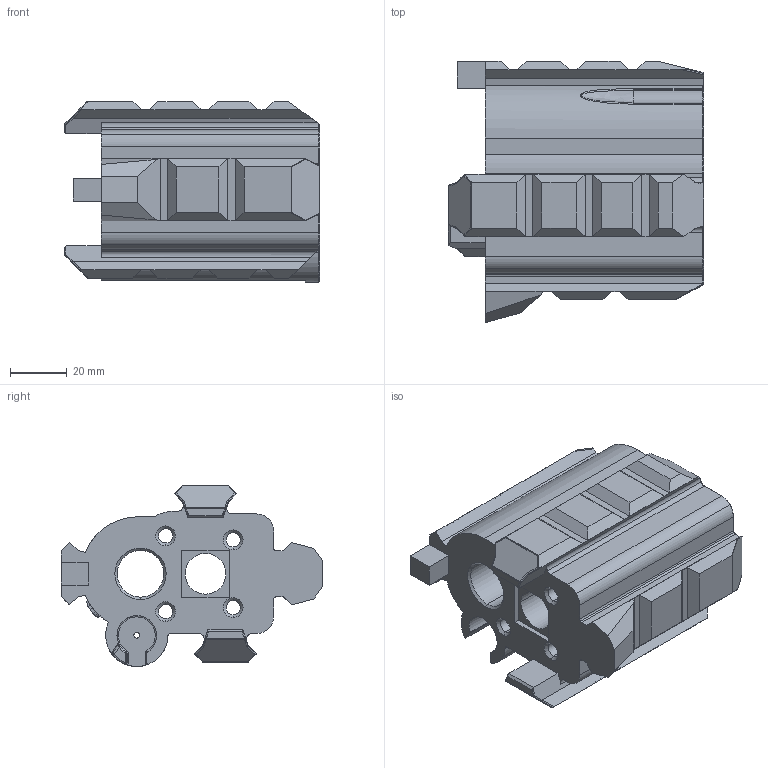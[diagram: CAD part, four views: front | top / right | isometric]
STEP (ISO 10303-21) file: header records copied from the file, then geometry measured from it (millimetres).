
FILE_DESCRIPTION(('STEP AP214'),'1');
FILE_NAME('Mod9 Barrel Retainer Final.stp','2020-09-28T22:44:09',(' '),(' '),'Spatial InterOp 3D',' ',' ');
FILE_SCHEMA(('AUTOMOTIVE_DESIGN { 1 0 10303 214 1 1 1 1 }'));
Length unit declared in the file: metre
Products named in the file (1): ASM Body
Bounding box: 90.02 x 92.13 x 63.85 mm (x, y, z)
Volume: 160852.1 mm3; surface area: 46398.1 mm2
Topology: 1 solids, 1 shells, 591 faces, 1595 edges, 1008 vertices
Faces by surface type: cylinder 195, plane 189, bspline 116, cone 68, torus 15, sphere 8
Entity records: 20893 total; most frequent: CARTESIAN_POINT 6688, ORIENTED_EDGE 3182, DIRECTION 2667, EDGE_CURVE 1591, VERTEX_POINT 1008, AXIS2_PLACEMENT_3D 932, LINE 803, VECTOR 803
